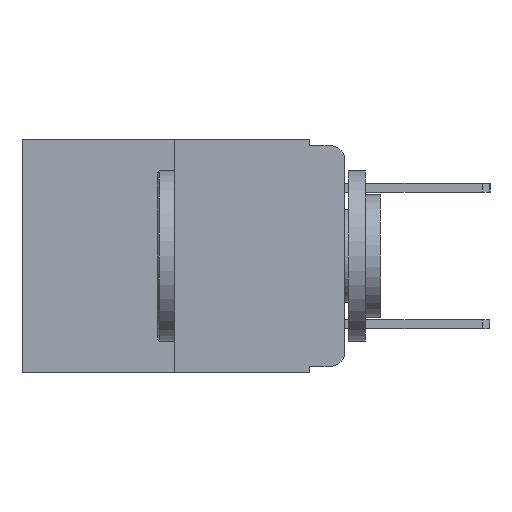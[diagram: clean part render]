
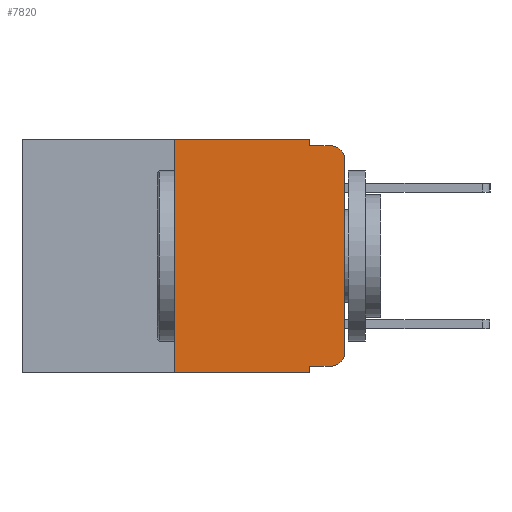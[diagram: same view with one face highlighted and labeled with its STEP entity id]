
A CAD part, left-side view. The second image highlights one B-rep face of the part: STEP entity #7820.
In plain terms, the highlighted planar face has unit normal (-1, 0, 0).
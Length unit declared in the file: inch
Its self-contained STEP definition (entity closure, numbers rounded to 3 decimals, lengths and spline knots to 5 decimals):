
#324 = VECTOR ( 'NONE', #13885, 39.37008 ) ;
#354 = EDGE_CURVE ( 'NONE', #13543, #10590, #13766, .T. ) ;
#438 = ORIENTED_EDGE ( 'NONE', *, *, #4770, .T. ) ;
#1074 = DIRECTION ( 'NONE',  ( 0., 0., -1. ) ) ;
#1775 = AXIS2_PLACEMENT_3D ( 'NONE', #6757, #14267, #7913 ) ;
#2049 = VECTOR ( 'NONE', #4438, 39.37008 ) ;
#2129 = VERTEX_POINT ( 'NONE', #12597 ) ;
#2146 = CIRCLE ( 'NONE', #1775, 0.02 ) ;
#2230 = DIRECTION ( 'NONE',  ( 0., -1., 0. ) ) ;
#2263 = CARTESIAN_POINT ( 'NONE',  ( 0., 0., -0.313 ) ) ;
#2586 = CARTESIAN_POINT ( 'NONE',  ( 0., 0.051, 0. ) ) ;
#2720 = CARTESIAN_POINT ( 'NONE',  ( 0., 0., 0. ) ) ;
#3161 = VECTOR ( 'NONE', #11887, 39.37008 ) ;
#3232 = EDGE_CURVE ( 'NONE', #3772, #6658, #5958, .T. ) ;
#3677 = VERTEX_POINT ( 'NONE', #2586 ) ;
#3772 = VERTEX_POINT ( 'NONE', #8808 ) ;
#3899 = CARTESIAN_POINT ( 'NONE',  ( 0., 0.02, -0.01 ) ) ;
#3911 = CARTESIAN_POINT ( 'NONE',  ( 0., 0.051, 0. ) ) ;
#4003 = EDGE_CURVE ( 'NONE', #10590, #3677, #9095, .T. ) ;
#4118 = ORIENTED_EDGE ( 'NONE', *, *, #4228, .T. ) ;
#4228 = EDGE_CURVE ( 'NONE', #3772, #2129, #7889, .T. ) ;
#4438 = DIRECTION ( 'NONE',  ( 0., 0., 1. ) ) ;
#4539 = DIRECTION ( 'NONE',  ( 1., 0., 0. ) ) ;
#4707 = EDGE_CURVE ( 'NONE', #2129, #10359, #8385, .T. ) ;
#4770 = EDGE_CURVE ( 'NONE', #6844, #5960, #2146, .T. ) ;
#4781 = VECTOR ( 'NONE', #9931, 39.37008 ) ;
#5401 = EDGE_CURVE ( 'NONE', #10359, #6844, #12532, .T. ) ;
#5492 = CARTESIAN_POINT ( 'NONE',  ( 0., 0., -0.03 ) ) ;
#5513 = CARTESIAN_POINT ( 'NONE',  ( 0., 0.25, 0. ) ) ;
#5595 = AXIS2_PLACEMENT_3D ( 'NONE', #10204, #4539, #12299 ) ;
#5958 = LINE ( 'NONE', #3911, #14233 ) ;
#5960 = VERTEX_POINT ( 'NONE', #3899 ) ;
#6557 = DIRECTION ( 'NONE',  ( -1., 0., 0. ) ) ;
#6658 = VERTEX_POINT ( 'NONE', #11868 ) ;
#6757 = CARTESIAN_POINT ( 'NONE',  ( 0., 0.02, -0.03 ) ) ;
#6844 = VERTEX_POINT ( 'NONE', #5492 ) ;
#7260 = FACE_OUTER_BOUND ( 'NONE', #13667, .T. ) ;
#7497 = CARTESIAN_POINT ( 'NONE',  ( 0., 0.25, 0. ) ) ;
#7499 = CARTESIAN_POINT ( 'NONE',  ( 0., 0.473, -0.343 ) ) ;
#7614 = ORIENTED_EDGE ( 'NONE', *, *, #11749, .F. ) ;
#7758 = LINE ( 'NONE', #14771, #10317 ) ;
#7820 = ADVANCED_FACE ( 'NONE', ( #7260 ), #14328, .F. ) ;
#7848 = AXIS2_PLACEMENT_3D ( 'NONE', #13010, #6557, #14078 ) ;
#7889 = LINE ( 'NONE', #14092, #4781 ) ;
#7913 = DIRECTION ( 'NONE',  ( 0., 0., -1. ) ) ;
#8170 = ORIENTED_EDGE ( 'NONE', *, *, #354, .F. ) ;
#8385 = CIRCLE ( 'NONE', #7848, 0.02 ) ;
#8434 = VERTEX_POINT ( 'NONE', #10840 ) ;
#8513 = VECTOR ( 'NONE', #2230, 39.37008 ) ;
#8662 = ORIENTED_EDGE ( 'NONE', *, *, #13917, .F. ) ;
#8808 = CARTESIAN_POINT ( 'NONE',  ( 0., 0.051, -0.333 ) ) ;
#8857 = ORIENTED_EDGE ( 'NONE', *, *, #3232, .F. ) ;
#9095 = LINE ( 'NONE', #12579, #11584 ) ;
#9669 = ORIENTED_EDGE ( 'NONE', *, *, #4003, .F. ) ;
#9931 = DIRECTION ( 'NONE',  ( 0., -1., 0. ) ) ;
#10162 = CARTESIAN_POINT ( 'NONE',  ( 0., 0.25, -0.343 ) ) ;
#10204 = CARTESIAN_POINT ( 'NONE',  ( 0., 0.473, 0. ) ) ;
#10317 = VECTOR ( 'NONE', #1074, 39.37008 ) ;
#10343 = LINE ( 'NONE', #7499, #324 ) ;
#10359 = VERTEX_POINT ( 'NONE', #2263 ) ;
#10590 = VERTEX_POINT ( 'NONE', #7497 ) ;
#10797 = DIRECTION ( 'NONE',  ( 0., 0., -1. ) ) ;
#10840 = CARTESIAN_POINT ( 'NONE',  ( 0., 0.051, -0.01 ) ) ;
#11358 = LINE ( 'NONE', #11453, #8513 ) ;
#11453 = CARTESIAN_POINT ( 'NONE',  ( 0., 0.051, -0.01 ) ) ;
#11540 = DIRECTION ( 'NONE',  ( 0., -1., 0. ) ) ;
#11557 = ORIENTED_EDGE ( 'NONE', *, *, #5401, .T. ) ;
#11584 = VECTOR ( 'NONE', #11540, 39.37008 ) ;
#11749 = EDGE_CURVE ( 'NONE', #8434, #5960, #11358, .T. ) ;
#11868 = CARTESIAN_POINT ( 'NONE',  ( 0., 0.051, -0.343 ) ) ;
#11887 = DIRECTION ( 'NONE',  ( 0., 0., 1. ) ) ;
#12151 = ORIENTED_EDGE ( 'NONE', *, *, #12617, .T. ) ;
#12299 = DIRECTION ( 'NONE',  ( 0., 0., -1. ) ) ;
#12532 = LINE ( 'NONE', #2720, #3161 ) ;
#12579 = CARTESIAN_POINT ( 'NONE',  ( 0., 0.473, 0. ) ) ;
#12597 = CARTESIAN_POINT ( 'NONE',  ( 0., 0.02, -0.333 ) ) ;
#12617 = EDGE_CURVE ( 'NONE', #13543, #6658, #10343, .T. ) ;
#13010 = CARTESIAN_POINT ( 'NONE',  ( 0., 0.02, -0.313 ) ) ;
#13543 = VERTEX_POINT ( 'NONE', #10162 ) ;
#13667 = EDGE_LOOP ( 'NONE', ( #11557, #438, #7614, #8662, #9669, #8170, #12151, #8857, #4118, #13962 ) ) ;
#13766 = LINE ( 'NONE', #5513, #2049 ) ;
#13885 = DIRECTION ( 'NONE',  ( 0., -1., 0. ) ) ;
#13917 = EDGE_CURVE ( 'NONE', #3677, #8434, #7758, .T. ) ;
#13962 = ORIENTED_EDGE ( 'NONE', *, *, #4707, .T. ) ;
#14078 = DIRECTION ( 'NONE',  ( 0., 0., -1. ) ) ;
#14092 = CARTESIAN_POINT ( 'NONE',  ( 0., 0.051, -0.333 ) ) ;
#14233 = VECTOR ( 'NONE', #10797, 39.37008 ) ;
#14267 = DIRECTION ( 'NONE',  ( -1., 0., 0. ) ) ;
#14328 = PLANE ( 'NONE',  #5595 ) ;
#14771 = CARTESIAN_POINT ( 'NONE',  ( 0., 0.051, 0. ) ) ;
